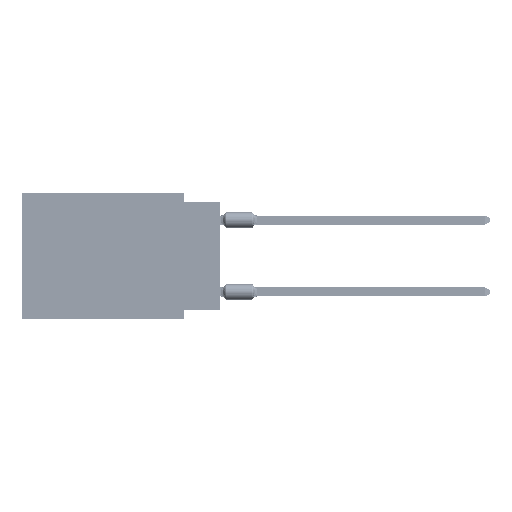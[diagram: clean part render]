
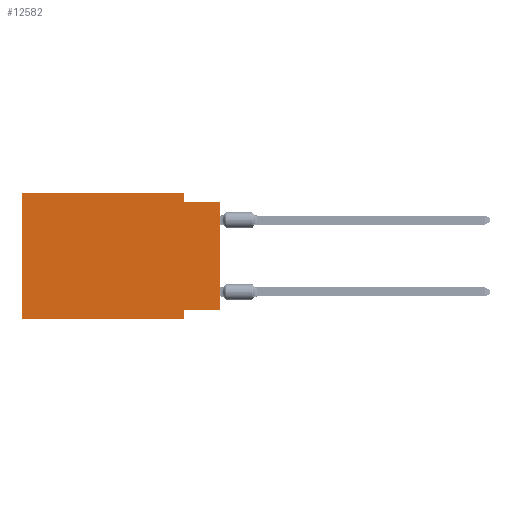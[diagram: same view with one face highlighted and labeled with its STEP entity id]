
A CAD part, left-side view. The second image highlights one B-rep face of the part: STEP entity #12582.
In plain terms, the highlighted planar face has unit normal (-1, 0, 0).
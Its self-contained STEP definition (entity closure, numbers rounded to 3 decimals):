
#368 = PLANE ( 'NONE',  #53359 ) ;
#3218 = CARTESIAN_POINT ( 'NONE',  ( 0., 2.54, -8.255 ) ) ;
#3688 = VECTOR ( 'NONE', #53931, 1000. ) ;
#3868 = CARTESIAN_POINT ( 'NONE',  ( 0., 0., -0.635 ) ) ;
#4323 = EDGE_CURVE ( 'NONE', #89639, #47717, #19798, .T. ) ;
#4928 = DIRECTION ( 'NONE',  ( 0., -1., 0. ) ) ;
#5266 = ORIENTED_EDGE ( 'NONE', *, *, #30885, .F. ) ;
#6466 = VECTOR ( 'NONE', #101043, 1000. ) ;
#6557 = VERTEX_POINT ( 'NONE', #70230 ) ;
#11537 = VERTEX_POINT ( 'NONE', #73633 ) ;
#12448 = DIRECTION ( 'NONE',  ( 0., 0., -1. ) ) ;
#12582 = ADVANCED_FACE ( 'NONE', ( #35088 ), #368, .F. ) ;
#15068 = VECTOR ( 'NONE', #99427, 1000. ) ;
#18555 = DIRECTION ( 'NONE',  ( 1., 0., 0. ) ) ;
#18629 = CARTESIAN_POINT ( 'NONE',  ( 0., 0., -8.255 ) ) ;
#19798 = LINE ( 'NONE', #20362, #46583 ) ;
#20362 = CARTESIAN_POINT ( 'NONE',  ( 0., 0., -8.255 ) ) ;
#20992 = CARTESIAN_POINT ( 'NONE',  ( 0., 2.54, -8.89 ) ) ;
#23449 = ORIENTED_EDGE ( 'NONE', *, *, #86795, .T. ) ;
#25820 = ORIENTED_EDGE ( 'NONE', *, *, #4323, .F. ) ;
#27865 = LINE ( 'NONE', #20992, #96773 ) ;
#30059 = CARTESIAN_POINT ( 'NONE',  ( 0., 13.97, 0. ) ) ;
#30877 = EDGE_CURVE ( 'NONE', #6557, #63519, #92030, .T. ) ;
#30885 = EDGE_CURVE ( 'NONE', #47100, #11537, #40258, .T. ) ;
#35088 = FACE_OUTER_BOUND ( 'NONE', #44721, .T. ) ;
#38281 = CARTESIAN_POINT ( 'NONE',  ( 0., 13.97, -8.89 ) ) ;
#38486 = ORIENTED_EDGE ( 'NONE', *, *, #99134, .T. ) ;
#40258 = LINE ( 'NONE', #30059, #15068 ) ;
#44683 = CARTESIAN_POINT ( 'NONE',  ( 0., 2.54, 0. ) ) ;
#44721 = EDGE_LOOP ( 'NONE', ( #23449, #88629, #94293, #65780, #5266, #38486, #99199, #25820 ) ) ;
#46583 = VECTOR ( 'NONE', #80122, 1000. ) ;
#47100 = VERTEX_POINT ( 'NONE', #38281 ) ;
#47717 = VERTEX_POINT ( 'NONE', #3218 ) ;
#52648 = DIRECTION ( 'NONE',  ( 0., 0., -1. ) ) ;
#53359 = AXIS2_PLACEMENT_3D ( 'NONE', #77190, #18555, #96480 ) ;
#53913 = LINE ( 'NONE', #108465, #68028 ) ;
#53931 = DIRECTION ( 'NONE',  ( 0., 0., 1. ) ) ;
#57887 = DIRECTION ( 'NONE',  ( 0., -1., 0. ) ) ;
#58615 = EDGE_CURVE ( 'NONE', #11537, #102815, #53913, .T. ) ;
#63519 = VERTEX_POINT ( 'NONE', #94935 ) ;
#65780 = ORIENTED_EDGE ( 'NONE', *, *, #58615, .F. ) ;
#65817 = CARTESIAN_POINT ( 'NONE',  ( 0., 13.97, -8.89 ) ) ;
#68028 = VECTOR ( 'NONE', #4928, 1000. ) ;
#70230 = CARTESIAN_POINT ( 'NONE',  ( 0., 2.54, -0.635 ) ) ;
#71980 = CARTESIAN_POINT ( 'NONE',  ( 0., 2.54, -8.89 ) ) ;
#72042 = EDGE_CURVE ( 'NONE', #102815, #6557, #89012, .T. ) ;
#73633 = CARTESIAN_POINT ( 'NONE',  ( 0., 13.97, 0. ) ) ;
#75920 = EDGE_CURVE ( 'NONE', #47717, #78999, #27865, .T. ) ;
#77190 = CARTESIAN_POINT ( 'NONE',  ( 0., 13.97, 0. ) ) ;
#78999 = VERTEX_POINT ( 'NONE', #71980 ) ;
#80122 = DIRECTION ( 'NONE',  ( 0., 1., 0. ) ) ;
#81034 = CARTESIAN_POINT ( 'NONE',  ( 0., 2.54, 0. ) ) ;
#86795 = EDGE_CURVE ( 'NONE', #89639, #63519, #105692, .T. ) ;
#88629 = ORIENTED_EDGE ( 'NONE', *, *, #30877, .F. ) ;
#89012 = LINE ( 'NONE', #44683, #89559 ) ;
#89182 = CARTESIAN_POINT ( 'NONE',  ( 0., 0., 0. ) ) ;
#89559 = VECTOR ( 'NONE', #52648, 1000. ) ;
#89639 = VERTEX_POINT ( 'NONE', #18629 ) ;
#92030 = LINE ( 'NONE', #3868, #109496 ) ;
#94293 = ORIENTED_EDGE ( 'NONE', *, *, #72042, .F. ) ;
#94935 = CARTESIAN_POINT ( 'NONE',  ( 0., 0., -0.635 ) ) ;
#96480 = DIRECTION ( 'NONE',  ( 0., 0., -1. ) ) ;
#96773 = VECTOR ( 'NONE', #12448, 1000. ) ;
#99134 = EDGE_CURVE ( 'NONE', #47100, #78999, #108463, .T. ) ;
#99199 = ORIENTED_EDGE ( 'NONE', *, *, #75920, .F. ) ;
#99427 = DIRECTION ( 'NONE',  ( 0., 0., 1. ) ) ;
#101043 = DIRECTION ( 'NONE',  ( 0., -1., 0. ) ) ;
#102815 = VERTEX_POINT ( 'NONE', #81034 ) ;
#105692 = LINE ( 'NONE', #89182, #3688 ) ;
#108463 = LINE ( 'NONE', #65817, #6466 ) ;
#108465 = CARTESIAN_POINT ( 'NONE',  ( 0., 13.97, 0. ) ) ;
#109496 = VECTOR ( 'NONE', #57887, 1000. ) ;
